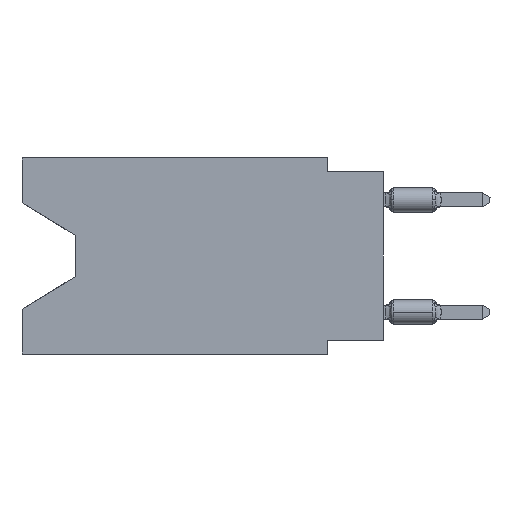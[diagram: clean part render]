
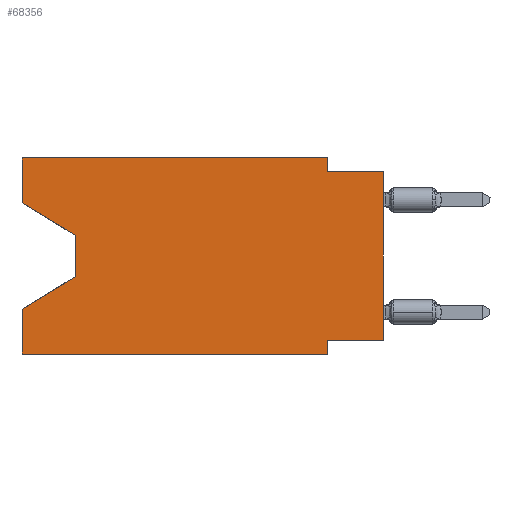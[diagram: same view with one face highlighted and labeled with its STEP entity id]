
A CAD part, left-side view. The second image highlights one B-rep face of the part: STEP entity #68356.
In plain terms, the highlighted planar face has unit normal (-1, 0, 0).
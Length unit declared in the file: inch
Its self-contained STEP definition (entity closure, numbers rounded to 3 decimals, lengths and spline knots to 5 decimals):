
#450 = VERTEX_POINT ( 'NONE', #56286 ) ;
#808 = CARTESIAN_POINT ( 'NONE',  ( 0., 0., -0.025 ) ) ;
#1892 = VECTOR ( 'NONE', #15469, 39.37008 ) ;
#1927 = ORIENTED_EDGE ( 'NONE', *, *, #30411, .T. ) ;
#2624 = CARTESIAN_POINT ( 'NONE',  ( 0., 0.55, -0.138 ) ) ;
#3251 = EDGE_CURVE ( 'NONE', #53888, #49231, #24625, .T. ) ;
#3752 = VECTOR ( 'NONE', #31347, 39.37008 ) ;
#4970 = VECTOR ( 'NONE', #69020, 39.37008 ) ;
#5401 = LINE ( 'NONE', #68014, #1892 ) ;
#8584 = CARTESIAN_POINT ( 'NONE',  ( 0., 0., -0.325 ) ) ;
#9354 = CARTESIAN_POINT ( 'NONE',  ( 0., 0.1, -0.325 ) ) ;
#10334 = DIRECTION ( 'NONE',  ( 0., 0., -1. ) ) ;
#11115 = CARTESIAN_POINT ( 'NONE',  ( 0., 0.1, -0.025 ) ) ;
#11394 = LINE ( 'NONE', #40107, #33417 ) ;
#13067 = CARTESIAN_POINT ( 'NONE',  ( 0., 0., -0.025 ) ) ;
#14553 = DIRECTION ( 'NONE',  ( 0., -1., 0. ) ) ;
#14818 = ORIENTED_EDGE ( 'NONE', *, *, #62542, .T. ) ;
#15469 = DIRECTION ( 'NONE',  ( 0., 0., -1. ) ) ;
#15795 = VERTEX_POINT ( 'NONE', #9354 ) ;
#16693 = CARTESIAN_POINT ( 'NONE',  ( 0., 0.645, 0. ) ) ;
#17124 = AXIS2_PLACEMENT_3D ( 'NONE', #21123, #27457, #10334 ) ;
#18201 = CARTESIAN_POINT ( 'NONE',  ( 0., 0., -0.325 ) ) ;
#18438 = CARTESIAN_POINT ( 'NONE',  ( 0., 0.645, -0.08025 ) ) ;
#20642 = ORIENTED_EDGE ( 'NONE', *, *, #61357, .F. ) ;
#21123 = CARTESIAN_POINT ( 'NONE',  ( 0., 0.645, 0. ) ) ;
#24625 = LINE ( 'NONE', #54118, #38772 ) ;
#24967 = DIRECTION ( 'NONE',  ( 0., 0., -1. ) ) ;
#25124 = VECTOR ( 'NONE', #44303, 39.37008 ) ;
#26739 = PLANE ( 'NONE',  #17124 ) ;
#26766 = VERTEX_POINT ( 'NONE', #32325 ) ;
#26829 = LINE ( 'NONE', #37678, #33232 ) ;
#27457 = DIRECTION ( 'NONE',  ( 1., 0., 0. ) ) ;
#27502 = EDGE_CURVE ( 'NONE', #49847, #41792, #26829, .T. ) ;
#27835 = CARTESIAN_POINT ( 'NONE',  ( 0., 0.645, 0. ) ) ;
#27863 = CARTESIAN_POINT ( 'NONE',  ( 0., 0.645, 0. ) ) ;
#28911 = ORIENTED_EDGE ( 'NONE', *, *, #3251, .T. ) ;
#28980 = VERTEX_POINT ( 'NONE', #13067 ) ;
#30411 = EDGE_CURVE ( 'NONE', #41216, #450, #42147, .T. ) ;
#30653 = ORIENTED_EDGE ( 'NONE', *, *, #62506, .F. ) ;
#31347 = DIRECTION ( 'NONE',  ( 0., 0., 1. ) ) ;
#32325 = CARTESIAN_POINT ( 'NONE',  ( 0., 0.645, -0.26975 ) ) ;
#33232 = VECTOR ( 'NONE', #14553, 39.37008 ) ;
#33396 = LINE ( 'NONE', #44607, #54484 ) ;
#33417 = VECTOR ( 'NONE', #62852, 39.37008 ) ;
#33606 = EDGE_CURVE ( 'NONE', #69283, #15795, #59668, .T. ) ;
#33816 = ORIENTED_EDGE ( 'NONE', *, *, #40498, .T. ) ;
#34121 = DIRECTION ( 'NONE',  ( 0., -0.855, -0.519 ) ) ;
#34505 = CARTESIAN_POINT ( 'NONE',  ( 0., 0.1, 0. ) ) ;
#34555 = ORIENTED_EDGE ( 'NONE', *, *, #37945, .T. ) ;
#34988 = VECTOR ( 'NONE', #36918, 39.37008 ) ;
#35437 = VECTOR ( 'NONE', #72574, 39.37008 ) ;
#36918 = DIRECTION ( 'NONE',  ( 0., 1., 0. ) ) ;
#37678 = CARTESIAN_POINT ( 'NONE',  ( 0., 0.645, 0. ) ) ;
#37797 = ORIENTED_EDGE ( 'NONE', *, *, #33606, .F. ) ;
#37945 = EDGE_CURVE ( 'NONE', #450, #26766, #33396, .T. ) ;
#38772 = VECTOR ( 'NONE', #53736, 39.37008 ) ;
#39735 = LINE ( 'NONE', #18438, #71720 ) ;
#40107 = CARTESIAN_POINT ( 'NONE',  ( 0., 0.1, -0.35 ) ) ;
#40498 = EDGE_CURVE ( 'NONE', #43353, #41216, #39735, .T. ) ;
#40792 = ORIENTED_EDGE ( 'NONE', *, *, #58889, .F. ) ;
#41182 = ORIENTED_EDGE ( 'NONE', *, *, #27502, .F. ) ;
#41216 = VERTEX_POINT ( 'NONE', #44428 ) ;
#41792 = VERTEX_POINT ( 'NONE', #34505 ) ;
#42147 = LINE ( 'NONE', #2624, #70501 ) ;
#42765 = VERTEX_POINT ( 'NONE', #11115 ) ;
#43353 = VERTEX_POINT ( 'NONE', #68414 ) ;
#44303 = DIRECTION ( 'NONE',  ( 0., 0., 1. ) ) ;
#44428 = CARTESIAN_POINT ( 'NONE',  ( 0., 0.55, -0.138 ) ) ;
#44607 = CARTESIAN_POINT ( 'NONE',  ( 0., 0.55, -0.212 ) ) ;
#48892 = EDGE_LOOP ( 'NONE', ( #33816, #1927, #34555, #66422, #28911, #20642, #37797, #14818, #30653, #58050, #41182, #40792 ) ) ;
#49143 = FACE_OUTER_BOUND ( 'NONE', #48892, .T. ) ;
#49225 = EDGE_CURVE ( 'NONE', #53888, #26766, #72270, .T. ) ;
#49231 = VERTEX_POINT ( 'NONE', #66669 ) ;
#49847 = VERTEX_POINT ( 'NONE', #27863 ) ;
#51887 = LINE ( 'NONE', #808, #4970 ) ;
#53736 = DIRECTION ( 'NONE',  ( 0., -1., 0. ) ) ;
#53888 = VERTEX_POINT ( 'NONE', #53894 ) ;
#53894 = CARTESIAN_POINT ( 'NONE',  ( 0., 0.645, -0.35 ) ) ;
#54118 = CARTESIAN_POINT ( 'NONE',  ( 0., 0.645, -0.35 ) ) ;
#54484 = VECTOR ( 'NONE', #55439, 39.37008 ) ;
#55439 = DIRECTION ( 'NONE',  ( 0., 0.855, -0.519 ) ) ;
#56286 = CARTESIAN_POINT ( 'NONE',  ( 0., 0.55, -0.212 ) ) ;
#58050 = ORIENTED_EDGE ( 'NONE', *, *, #72734, .F. ) ;
#58889 = EDGE_CURVE ( 'NONE', #43353, #49847, #60049, .T. ) ;
#59668 = LINE ( 'NONE', #8584, #34988 ) ;
#60049 = LINE ( 'NONE', #27835, #35437 ) ;
#61357 = EDGE_CURVE ( 'NONE', #15795, #49231, #11394, .T. ) ;
#62506 = EDGE_CURVE ( 'NONE', #42765, #28980, #51887, .T. ) ;
#62542 = EDGE_CURVE ( 'NONE', #69283, #28980, #65281, .T. ) ;
#62852 = DIRECTION ( 'NONE',  ( 0., 0., -1. ) ) ;
#64558 = CARTESIAN_POINT ( 'NONE',  ( 0., 0., 0. ) ) ;
#65281 = LINE ( 'NONE', #64558, #3752 ) ;
#66422 = ORIENTED_EDGE ( 'NONE', *, *, #49225, .F. ) ;
#66669 = CARTESIAN_POINT ( 'NONE',  ( 0., 0.1, -0.35 ) ) ;
#68014 = CARTESIAN_POINT ( 'NONE',  ( 0., 0.1, 0. ) ) ;
#68356 = ADVANCED_FACE ( 'NONE', ( #49143 ), #26739, .F. ) ;
#68414 = CARTESIAN_POINT ( 'NONE',  ( 0., 0.645, -0.08025 ) ) ;
#69020 = DIRECTION ( 'NONE',  ( 0., -1., 0. ) ) ;
#69283 = VERTEX_POINT ( 'NONE', #18201 ) ;
#70501 = VECTOR ( 'NONE', #24967, 39.37008 ) ;
#71720 = VECTOR ( 'NONE', #34121, 39.37008 ) ;
#72270 = LINE ( 'NONE', #16693, #25124 ) ;
#72574 = DIRECTION ( 'NONE',  ( 0., 0., 1. ) ) ;
#72734 = EDGE_CURVE ( 'NONE', #41792, #42765, #5401, .T. ) ;
